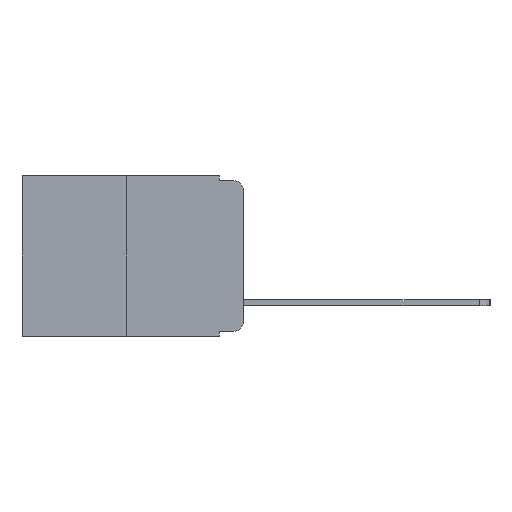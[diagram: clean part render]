
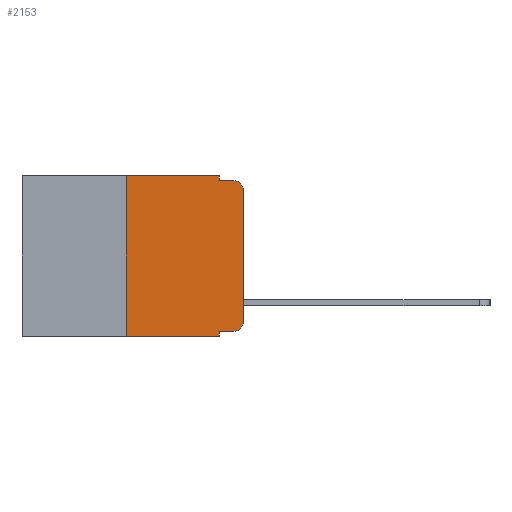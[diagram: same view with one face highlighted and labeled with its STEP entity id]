
A CAD part, left-side view. The second image highlights one B-rep face of the part: STEP entity #2153.
In plain terms, the highlighted planar face has unit normal (-1, 0, 0).
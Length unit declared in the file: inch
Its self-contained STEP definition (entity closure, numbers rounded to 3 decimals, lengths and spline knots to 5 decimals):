
#114 = ORIENTED_EDGE ( 'NONE', *, *, #9587, .F. ) ;
#341 = CARTESIAN_POINT ( 'NONE',  ( 0., 0.051, 0. ) ) ;
#458 = ORIENTED_EDGE ( 'NONE', *, *, #5536, .F. ) ;
#620 = EDGE_CURVE ( 'NONE', #14693, #11029, #3768, .T. ) ;
#794 = AXIS2_PLACEMENT_3D ( 'NONE', #15438, #8059, #16665 ) ;
#911 = EDGE_CURVE ( 'NONE', #4061, #5297, #16507, .T. ) ;
#1401 = CARTESIAN_POINT ( 'NONE',  ( 0., 0., -0.03 ) ) ;
#1694 = EDGE_CURVE ( 'NONE', #8873, #14693, #14557, .T. ) ;
#1852 = VECTOR ( 'NONE', #5881, 39.37008 ) ;
#1913 = CARTESIAN_POINT ( 'NONE',  ( 0., 0., 0. ) ) ;
#1916 = ORIENTED_EDGE ( 'NONE', *, *, #911, .T. ) ;
#1976 = DIRECTION ( 'NONE',  ( 0., 0., 1. ) ) ;
#2141 = DIRECTION ( 'NONE',  ( 0., 0., -1. ) ) ;
#2153 = ADVANCED_FACE ( 'NONE', ( #4914 ), #10706, .F. ) ;
#2877 = DIRECTION ( 'NONE',  ( 0., 0., -1. ) ) ;
#3212 = LINE ( 'NONE', #341, #16445 ) ;
#3459 = DIRECTION ( 'NONE',  ( 0., 0., -1. ) ) ;
#3490 = DIRECTION ( 'NONE',  ( 0., -1., 0. ) ) ;
#3633 = CARTESIAN_POINT ( 'NONE',  ( 0., 0.051, -0.333 ) ) ;
#3703 = EDGE_CURVE ( 'NONE', #8873, #5297, #3985, .T. ) ;
#3768 = CIRCLE ( 'NONE', #12209, 0.02 ) ;
#3985 = LINE ( 'NONE', #10933, #11037 ) ;
#4045 = CARTESIAN_POINT ( 'NONE',  ( 0., 0.051, 0. ) ) ;
#4061 = VERTEX_POINT ( 'NONE', #13176 ) ;
#4651 = EDGE_CURVE ( 'NONE', #4061, #15427, #5245, .T. ) ;
#4709 = CARTESIAN_POINT ( 'NONE',  ( 0., 0.051, -0.333 ) ) ;
#4914 = FACE_OUTER_BOUND ( 'NONE', #12560, .T. ) ;
#5081 = ORIENTED_EDGE ( 'NONE', *, *, #620, .T. ) ;
#5245 = LINE ( 'NONE', #9895, #1852 ) ;
#5297 = VERTEX_POINT ( 'NONE', #8560 ) ;
#5536 = EDGE_CURVE ( 'NONE', #15299, #8342, #3212, .T. ) ;
#5881 = DIRECTION ( 'NONE',  ( 0., 0., 1. ) ) ;
#6024 = ORIENTED_EDGE ( 'NONE', *, *, #4651, .F. ) ;
#6365 = ORIENTED_EDGE ( 'NONE', *, *, #1694, .T. ) ;
#6449 = EDGE_CURVE ( 'NONE', #8342, #13173, #16595, .T. ) ;
#6585 = ORIENTED_EDGE ( 'NONE', *, *, #8274, .T. ) ;
#6683 = ORIENTED_EDGE ( 'NONE', *, *, #7400, .T. ) ;
#6888 = DIRECTION ( 'NONE',  ( 0., 0., -1. ) ) ;
#6998 = DIRECTION ( 'NONE',  ( 1., 0., 0. ) ) ;
#7239 = ORIENTED_EDGE ( 'NONE', *, *, #6449, .F. ) ;
#7310 = CIRCLE ( 'NONE', #794, 0.02 ) ;
#7400 = EDGE_CURVE ( 'NONE', #9507, #13173, #7310, .T. ) ;
#7407 = CARTESIAN_POINT ( 'NONE',  ( 0., 0.25, 0. ) ) ;
#7911 = CARTESIAN_POINT ( 'NONE',  ( 0., 0.02, -0.01 ) ) ;
#8059 = DIRECTION ( 'NONE',  ( -1., 0., 0. ) ) ;
#8274 = EDGE_CURVE ( 'NONE', #11029, #9507, #12797, .T. ) ;
#8321 = ORIENTED_EDGE ( 'NONE', *, *, #3703, .F. ) ;
#8342 = VERTEX_POINT ( 'NONE', #11481 ) ;
#8560 = CARTESIAN_POINT ( 'NONE',  ( 0., 0.051, -0.343 ) ) ;
#8873 = VERTEX_POINT ( 'NONE', #4709 ) ;
#9321 = VECTOR ( 'NONE', #15883, 39.37008 ) ;
#9507 = VERTEX_POINT ( 'NONE', #1401 ) ;
#9547 = VECTOR ( 'NONE', #1976, 39.37008 ) ;
#9587 = EDGE_CURVE ( 'NONE', #15427, #15299, #15791, .T. ) ;
#9706 = CARTESIAN_POINT ( 'NONE',  ( 0., 0.473, -0.343 ) ) ;
#9740 = CARTESIAN_POINT ( 'NONE',  ( 0., 0.02, -0.333 ) ) ;
#9895 = CARTESIAN_POINT ( 'NONE',  ( 0., 0.25, 0. ) ) ;
#9909 = CARTESIAN_POINT ( 'NONE',  ( 0., 0.02, -0.313 ) ) ;
#10043 = VECTOR ( 'NONE', #12801, 39.37008 ) ;
#10498 = CARTESIAN_POINT ( 'NONE',  ( 0., 0., -0.313 ) ) ;
#10584 = DIRECTION ( 'NONE',  ( 0., -1., 0. ) ) ;
#10706 = PLANE ( 'NONE',  #16745 ) ;
#10933 = CARTESIAN_POINT ( 'NONE',  ( 0., 0.051, 0. ) ) ;
#11029 = VERTEX_POINT ( 'NONE', #10498 ) ;
#11037 = VECTOR ( 'NONE', #2877, 39.37008 ) ;
#11080 = CARTESIAN_POINT ( 'NONE',  ( 0., 0.473, 0. ) ) ;
#11375 = VECTOR ( 'NONE', #3490, 39.37008 ) ;
#11435 = CARTESIAN_POINT ( 'NONE',  ( 0., 0.473, 0. ) ) ;
#11481 = CARTESIAN_POINT ( 'NONE',  ( 0., 0.051, -0.01 ) ) ;
#12209 = AXIS2_PLACEMENT_3D ( 'NONE', #9909, #12246, #2141 ) ;
#12246 = DIRECTION ( 'NONE',  ( -1., 0., 0. ) ) ;
#12560 = EDGE_LOOP ( 'NONE', ( #6585, #6683, #7239, #458, #114, #6024, #1916, #8321, #6365, #5081 ) ) ;
#12797 = LINE ( 'NONE', #1913, #9547 ) ;
#12801 = DIRECTION ( 'NONE',  ( 0., -1., 0. ) ) ;
#12996 = VECTOR ( 'NONE', #10584, 39.37008 ) ;
#13173 = VERTEX_POINT ( 'NONE', #7911 ) ;
#13176 = CARTESIAN_POINT ( 'NONE',  ( 0., 0.25, -0.343 ) ) ;
#14557 = LINE ( 'NONE', #3633, #11375 ) ;
#14693 = VERTEX_POINT ( 'NONE', #9740 ) ;
#15299 = VERTEX_POINT ( 'NONE', #4045 ) ;
#15427 = VERTEX_POINT ( 'NONE', #7407 ) ;
#15438 = CARTESIAN_POINT ( 'NONE',  ( 0., 0.02, -0.03 ) ) ;
#15791 = LINE ( 'NONE', #11080, #9321 ) ;
#15883 = DIRECTION ( 'NONE',  ( 0., -1., 0. ) ) ;
#16445 = VECTOR ( 'NONE', #3459, 39.37008 ) ;
#16507 = LINE ( 'NONE', #9706, #10043 ) ;
#16595 = LINE ( 'NONE', #16609, #12996 ) ;
#16609 = CARTESIAN_POINT ( 'NONE',  ( 0., 0.051, -0.01 ) ) ;
#16665 = DIRECTION ( 'NONE',  ( 0., 0., -1. ) ) ;
#16745 = AXIS2_PLACEMENT_3D ( 'NONE', #11435, #6998, #6888 ) ;
